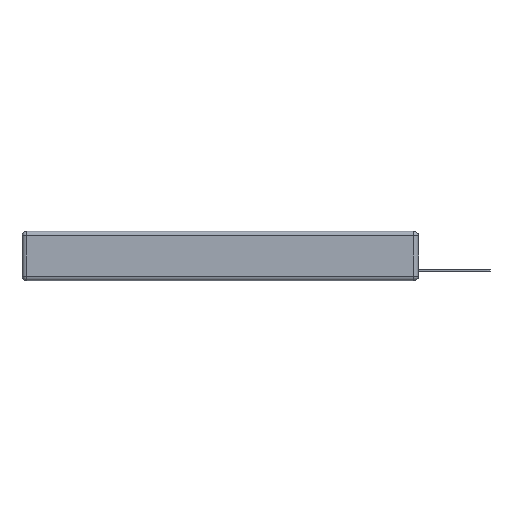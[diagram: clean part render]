
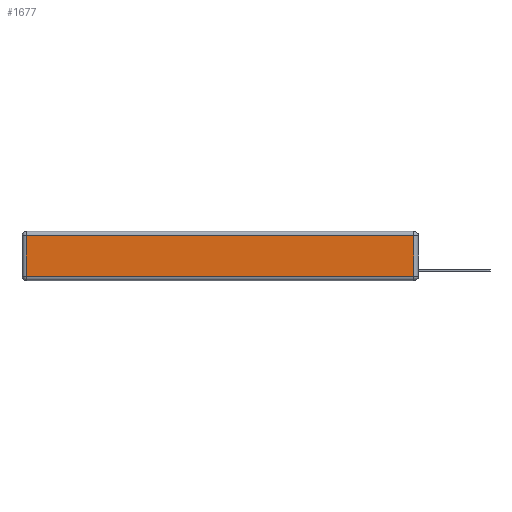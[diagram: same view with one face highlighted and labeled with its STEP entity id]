
A CAD part, left-side view. The second image highlights one B-rep face of the part: STEP entity #1677.
In plain terms, the highlighted planar face has unit normal (-1, 0, 0).
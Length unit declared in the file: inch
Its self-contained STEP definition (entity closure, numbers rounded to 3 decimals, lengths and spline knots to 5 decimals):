
#218 = DIRECTION ( 'NONE',  ( 0., 0., 1. ) ) ;
#670 = CARTESIAN_POINT ( 'NONE',  ( 0., 0.03, -0.343 ) ) ;
#840 = LINE ( 'NONE', #6411, #6320 ) ;
#857 = VECTOR ( 'NONE', #5221, 39.37008 ) ;
#1115 = CARTESIAN_POINT ( 'NONE',  ( 0., 2.75, -0.03 ) ) ;
#1204 = VERTEX_POINT ( 'NONE', #12269 ) ;
#1677 = ADVANCED_FACE ( 'NONE', ( #9792 ), #3948, .T. ) ;
#1919 = CARTESIAN_POINT ( 'NONE',  ( 0., 0., -0.313 ) ) ;
#2029 = ORIENTED_EDGE ( 'NONE', *, *, #7208, .T. ) ;
#2689 = LINE ( 'NONE', #670, #7436 ) ;
#3487 = LINE ( 'NONE', #1115, #857 ) ;
#3700 = EDGE_LOOP ( 'NONE', ( #10448, #8168, #2029, #11393 ) ) ;
#3948 = PLANE ( 'NONE',  #8442 ) ;
#4172 = LINE ( 'NONE', #1919, #11952 ) ;
#4939 = VERTEX_POINT ( 'NONE', #8308 ) ;
#4975 = CARTESIAN_POINT ( 'NONE',  ( 0., 0., -0.343 ) ) ;
#5221 = DIRECTION ( 'NONE',  ( 0., 1., 0. ) ) ;
#5386 = EDGE_CURVE ( 'NONE', #4939, #5483, #4172, .T. ) ;
#5483 = VERTEX_POINT ( 'NONE', #9137 ) ;
#6320 = VECTOR ( 'NONE', #9351, 39.37008 ) ;
#6411 = CARTESIAN_POINT ( 'NONE',  ( 0., 2.72, -0.343 ) ) ;
#7208 = EDGE_CURVE ( 'NONE', #7363, #1204, #3487, .T. ) ;
#7363 = VERTEX_POINT ( 'NONE', #10400 ) ;
#7436 = VECTOR ( 'NONE', #9949, 39.37008 ) ;
#8168 = ORIENTED_EDGE ( 'NONE', *, *, #8182, .T. ) ;
#8182 = EDGE_CURVE ( 'NONE', #5483, #7363, #2689, .T. ) ;
#8308 = CARTESIAN_POINT ( 'NONE',  ( 0., 2.72, -0.313 ) ) ;
#8442 = AXIS2_PLACEMENT_3D ( 'NONE', #4975, #9287, #218 ) ;
#9137 = CARTESIAN_POINT ( 'NONE',  ( 0., 0.03, -0.313 ) ) ;
#9287 = DIRECTION ( 'NONE',  ( -1., 0., 0. ) ) ;
#9351 = DIRECTION ( 'NONE',  ( 0., 0., -1. ) ) ;
#9792 = FACE_OUTER_BOUND ( 'NONE', #3700, .T. ) ;
#9949 = DIRECTION ( 'NONE',  ( 0., 0., 1. ) ) ;
#10400 = CARTESIAN_POINT ( 'NONE',  ( 0., 0.03, -0.03 ) ) ;
#10448 = ORIENTED_EDGE ( 'NONE', *, *, #5386, .T. ) ;
#11016 = DIRECTION ( 'NONE',  ( 0., -1., 0. ) ) ;
#11393 = ORIENTED_EDGE ( 'NONE', *, *, #12708, .T. ) ;
#11952 = VECTOR ( 'NONE', #11016, 39.37008 ) ;
#12269 = CARTESIAN_POINT ( 'NONE',  ( 0., 2.72, -0.03 ) ) ;
#12708 = EDGE_CURVE ( 'NONE', #1204, #4939, #840, .T. ) ;
